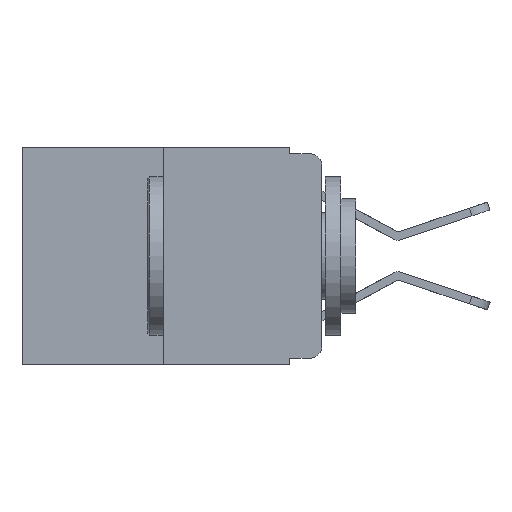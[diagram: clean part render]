
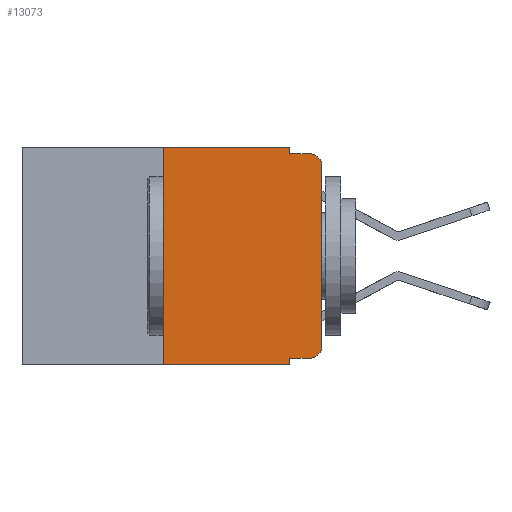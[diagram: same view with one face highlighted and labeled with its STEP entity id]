
A CAD part, left-side view. The second image highlights one B-rep face of the part: STEP entity #13073.
In plain terms, the highlighted planar face has unit normal (-1, 0, 0).
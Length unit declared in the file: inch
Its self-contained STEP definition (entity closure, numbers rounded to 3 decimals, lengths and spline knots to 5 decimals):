
#34 = VECTOR ( 'NONE', #18497, 39.37008 ) ;
#196 = CARTESIAN_POINT ( 'NONE',  ( 0., 0.473, 0. ) ) ;
#300 = LINE ( 'NONE', #13485, #4865 ) ;
#531 = DIRECTION ( 'NONE',  ( 0., 0., -1. ) ) ;
#550 = CARTESIAN_POINT ( 'NONE',  ( 0., 0.02, -0.03 ) ) ;
#825 = AXIS2_PLACEMENT_3D ( 'NONE', #1932, #15300, #531 ) ;
#1144 = EDGE_CURVE ( 'NONE', #11531, #7755, #17190, .T. ) ;
#1932 = CARTESIAN_POINT ( 'NONE',  ( 0., 0.473, 0. ) ) ;
#2008 = EDGE_CURVE ( 'NONE', #12175, #5640, #6656, .T. ) ;
#2305 = CARTESIAN_POINT ( 'NONE',  ( 0., 0., 0. ) ) ;
#2366 = AXIS2_PLACEMENT_3D ( 'NONE', #550, #16825, #13730 ) ;
#2489 = CARTESIAN_POINT ( 'NONE',  ( 0., 0.02, -0.333 ) ) ;
#2639 = CARTESIAN_POINT ( 'NONE',  ( 0., 0.25, -0.343 ) ) ;
#3168 = CIRCLE ( 'NONE', #19752, 0.02 ) ;
#3653 = LINE ( 'NONE', #10011, #17003 ) ;
#3867 = ORIENTED_EDGE ( 'NONE', *, *, #1144, .T. ) ;
#4037 = VERTEX_POINT ( 'NONE', #2489 ) ;
#4135 = ORIENTED_EDGE ( 'NONE', *, *, #6242, .F. ) ;
#4573 = CARTESIAN_POINT ( 'NONE',  ( 0., 0., -0.313 ) ) ;
#4583 = CARTESIAN_POINT ( 'NONE',  ( 0., 0., -0.03 ) ) ;
#4681 = CARTESIAN_POINT ( 'NONE',  ( 0., 0.02, -0.313 ) ) ;
#4789 = ORIENTED_EDGE ( 'NONE', *, *, #10529, .T. ) ;
#4865 = VECTOR ( 'NONE', #18863, 39.37008 ) ;
#5178 = CARTESIAN_POINT ( 'NONE',  ( 0., 0.02, -0.01 ) ) ;
#5224 = CARTESIAN_POINT ( 'NONE',  ( 0., 0.051, -0.333 ) ) ;
#5640 = VERTEX_POINT ( 'NONE', #16324 ) ;
#5643 = DIRECTION ( 'NONE',  ( 0., -1., 0. ) ) ;
#5722 = ORIENTED_EDGE ( 'NONE', *, *, #13101, .F. ) ;
#5760 = CARTESIAN_POINT ( 'NONE',  ( 0., 0.051, -0.343 ) ) ;
#5850 = LINE ( 'NONE', #8860, #20036 ) ;
#6242 = EDGE_CURVE ( 'NONE', #16286, #7755, #300, .T. ) ;
#6656 = LINE ( 'NONE', #196, #19956 ) ;
#6909 = EDGE_CURVE ( 'NONE', #4037, #20485, #3168, .T. ) ;
#6962 = LINE ( 'NONE', #2305, #8318 ) ;
#7755 = VERTEX_POINT ( 'NONE', #5178 ) ;
#8318 = VECTOR ( 'NONE', #8561, 39.37008 ) ;
#8396 = DIRECTION ( 'NONE',  ( 0., 0., 1. ) ) ;
#8550 = CARTESIAN_POINT ( 'NONE',  ( 0., 0.051, 0. ) ) ;
#8561 = DIRECTION ( 'NONE',  ( 0., 0., 1. ) ) ;
#8568 = ORIENTED_EDGE ( 'NONE', *, *, #2008, .F. ) ;
#8709 = PLANE ( 'NONE',  #825 ) ;
#8860 = CARTESIAN_POINT ( 'NONE',  ( 0., 0.473, -0.343 ) ) ;
#9870 = LINE ( 'NONE', #8550, #11143 ) ;
#10011 = CARTESIAN_POINT ( 'NONE',  ( 0., 0.25, 0. ) ) ;
#10529 = EDGE_CURVE ( 'NONE', #12450, #13864, #5850, .T. ) ;
#10856 = ORIENTED_EDGE ( 'NONE', *, *, #6909, .T. ) ;
#10914 = EDGE_CURVE ( 'NONE', #17437, #4037, #11983, .T. ) ;
#11143 = VECTOR ( 'NONE', #18179, 39.37008 ) ;
#11531 = VERTEX_POINT ( 'NONE', #4583 ) ;
#11983 = LINE ( 'NONE', #14227, #20056 ) ;
#12066 = FACE_OUTER_BOUND ( 'NONE', #21113, .T. ) ;
#12175 = VERTEX_POINT ( 'NONE', #19954 ) ;
#12450 = VERTEX_POINT ( 'NONE', #2639 ) ;
#13073 = ADVANCED_FACE ( 'NONE', ( #12066 ), #8709, .F. ) ;
#13101 = EDGE_CURVE ( 'NONE', #12450, #12175, #3653, .T. ) ;
#13485 = CARTESIAN_POINT ( 'NONE',  ( 0., 0.051, -0.01 ) ) ;
#13730 = DIRECTION ( 'NONE',  ( 0., 0., -1. ) ) ;
#13864 = VERTEX_POINT ( 'NONE', #5760 ) ;
#14227 = CARTESIAN_POINT ( 'NONE',  ( 0., 0.051, -0.333 ) ) ;
#14791 = ORIENTED_EDGE ( 'NONE', *, *, #20220, .T. ) ;
#15071 = DIRECTION ( 'NONE',  ( 0., -1., 0. ) ) ;
#15129 = EDGE_CURVE ( 'NONE', #17437, #13864, #18081, .T. ) ;
#15300 = DIRECTION ( 'NONE',  ( 1., 0., 0. ) ) ;
#16111 = ORIENTED_EDGE ( 'NONE', *, *, #10914, .T. ) ;
#16286 = VERTEX_POINT ( 'NONE', #19664 ) ;
#16324 = CARTESIAN_POINT ( 'NONE',  ( 0., 0.051, 0. ) ) ;
#16825 = DIRECTION ( 'NONE',  ( -1., 0., 0. ) ) ;
#17003 = VECTOR ( 'NONE', #8396, 39.37008 ) ;
#17190 = CIRCLE ( 'NONE', #2366, 0.02 ) ;
#17263 = EDGE_CURVE ( 'NONE', #5640, #16286, #9870, .T. ) ;
#17437 = VERTEX_POINT ( 'NONE', #5224 ) ;
#17839 = DIRECTION ( 'NONE',  ( -1., 0., 0. ) ) ;
#18081 = LINE ( 'NONE', #19939, #34 ) ;
#18179 = DIRECTION ( 'NONE',  ( 0., 0., -1. ) ) ;
#18497 = DIRECTION ( 'NONE',  ( 0., 0., -1. ) ) ;
#18863 = DIRECTION ( 'NONE',  ( 0., -1., 0. ) ) ;
#19148 = ORIENTED_EDGE ( 'NONE', *, *, #17263, .F. ) ;
#19261 = DIRECTION ( 'NONE',  ( 0., 0., -1. ) ) ;
#19664 = CARTESIAN_POINT ( 'NONE',  ( 0., 0.051, -0.01 ) ) ;
#19752 = AXIS2_PLACEMENT_3D ( 'NONE', #4681, #17839, #19261 ) ;
#19939 = CARTESIAN_POINT ( 'NONE',  ( 0., 0.051, 0. ) ) ;
#19954 = CARTESIAN_POINT ( 'NONE',  ( 0., 0.25, 0. ) ) ;
#19956 = VECTOR ( 'NONE', #15071, 39.37008 ) ;
#20036 = VECTOR ( 'NONE', #5643, 39.37008 ) ;
#20056 = VECTOR ( 'NONE', #20313, 39.37008 ) ;
#20220 = EDGE_CURVE ( 'NONE', #20485, #11531, #6962, .T. ) ;
#20313 = DIRECTION ( 'NONE',  ( 0., -1., 0. ) ) ;
#20485 = VERTEX_POINT ( 'NONE', #4573 ) ;
#21113 = EDGE_LOOP ( 'NONE', ( #14791, #3867, #4135, #19148, #8568, #5722, #4789, #21284, #16111, #10856 ) ) ;
#21284 = ORIENTED_EDGE ( 'NONE', *, *, #15129, .F. ) ;
